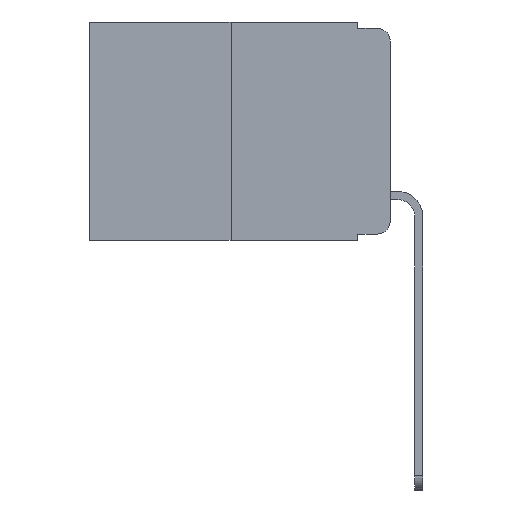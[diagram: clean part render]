
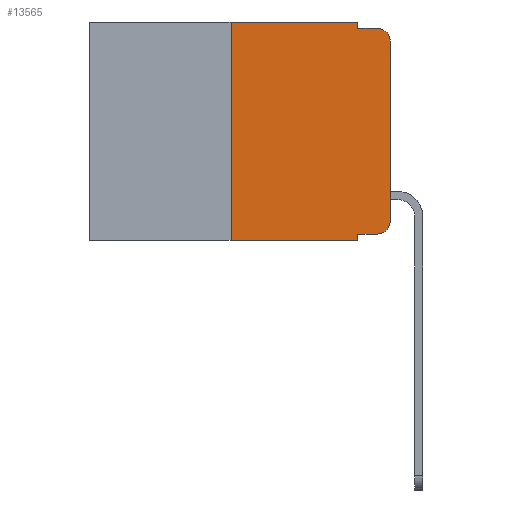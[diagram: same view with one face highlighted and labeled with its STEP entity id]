
A CAD part, left-side view. The second image highlights one B-rep face of the part: STEP entity #13565.
In plain terms, the highlighted planar face has unit normal (-1, 0, 0).
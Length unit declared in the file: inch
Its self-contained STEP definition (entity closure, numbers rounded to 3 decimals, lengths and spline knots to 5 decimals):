
#200 = EDGE_CURVE ( 'NONE', #16127, #12998, #8034, .T. ) ;
#222 = AXIS2_PLACEMENT_3D ( 'NONE', #17483, #13015, #17306 ) ;
#324 = ORIENTED_EDGE ( 'NONE', *, *, #8914, .T. ) ;
#459 = VECTOR ( 'NONE', #4900, 39.37008 ) ;
#764 = ORIENTED_EDGE ( 'NONE', *, *, #16925, .F. ) ;
#1282 = EDGE_CURVE ( 'NONE', #5609, #7590, #9548, .T. ) ;
#1350 = DIRECTION ( 'NONE',  ( 0., 0., -1. ) ) ;
#1611 = ORIENTED_EDGE ( 'NONE', *, *, #16746, .F. ) ;
#1637 = CARTESIAN_POINT ( 'NONE',  ( 0., 0.02, -0.313 ) ) ;
#1811 = VECTOR ( 'NONE', #4530, 39.37008 ) ;
#1812 = ORIENTED_EDGE ( 'NONE', *, *, #15690, .F. ) ;
#2113 = CIRCLE ( 'NONE', #18376, 0.02 ) ;
#3090 = VECTOR ( 'NONE', #7911, 39.37008 ) ;
#3169 = PLANE ( 'NONE',  #16164 ) ;
#3300 = EDGE_CURVE ( 'NONE', #13375, #14258, #11208, .T. ) ;
#3747 = VECTOR ( 'NONE', #1350, 39.37008 ) ;
#4145 = EDGE_CURVE ( 'NONE', #5609, #15441, #12513, .T. ) ;
#4530 = DIRECTION ( 'NONE',  ( 0., -1., 0. ) ) ;
#4900 = DIRECTION ( 'NONE',  ( 0., 0., 1. ) ) ;
#5467 = DIRECTION ( 'NONE',  ( 0., -1., 0. ) ) ;
#5485 = DIRECTION ( 'NONE',  ( 0., -1., 0. ) ) ;
#5609 = VERTEX_POINT ( 'NONE', #14676 ) ;
#5789 = CARTESIAN_POINT ( 'NONE',  ( 0., 0.051, -0.333 ) ) ;
#5985 = VERTEX_POINT ( 'NONE', #17091 ) ;
#6039 = CIRCLE ( 'NONE', #222, 0.02 ) ;
#6047 = CARTESIAN_POINT ( 'NONE',  ( 0., 0.473, 0. ) ) ;
#6854 = FACE_OUTER_BOUND ( 'NONE', #14925, .T. ) ;
#7193 = ORIENTED_EDGE ( 'NONE', *, *, #200, .T. ) ;
#7463 = ORIENTED_EDGE ( 'NONE', *, *, #4145, .T. ) ;
#7585 = CARTESIAN_POINT ( 'NONE',  ( 0., 0.25, 0. ) ) ;
#7590 = VERTEX_POINT ( 'NONE', #17943 ) ;
#7911 = DIRECTION ( 'NONE',  ( 0., -1., 0. ) ) ;
#8034 = LINE ( 'NONE', #16180, #459 ) ;
#8217 = VECTOR ( 'NONE', #11835, 39.37008 ) ;
#8445 = LINE ( 'NONE', #9388, #3090 ) ;
#8742 = CARTESIAN_POINT ( 'NONE',  ( 0., 0.051, -0.333 ) ) ;
#8914 = EDGE_CURVE ( 'NONE', #14258, #16127, #2113, .T. ) ;
#8921 = DIRECTION ( 'NONE',  ( 0., 0., -1. ) ) ;
#9120 = CARTESIAN_POINT ( 'NONE',  ( 0., 0., -0.03 ) ) ;
#9388 = CARTESIAN_POINT ( 'NONE',  ( 0., 0.051, -0.01 ) ) ;
#9548 = LINE ( 'NONE', #7585, #8217 ) ;
#10880 = VERTEX_POINT ( 'NONE', #17866 ) ;
#11109 = EDGE_CURVE ( 'NONE', #12998, #5985, #6039, .T. ) ;
#11208 = LINE ( 'NONE', #5789, #1811 ) ;
#11218 = CARTESIAN_POINT ( 'NONE',  ( 0., 0.473, -0.343 ) ) ;
#11639 = ORIENTED_EDGE ( 'NONE', *, *, #3300, .T. ) ;
#11835 = DIRECTION ( 'NONE',  ( 0., 0., 1. ) ) ;
#12057 = CARTESIAN_POINT ( 'NONE',  ( 0., 0., -0.313 ) ) ;
#12318 = DIRECTION ( 'NONE',  ( 0., 0., -1. ) ) ;
#12513 = LINE ( 'NONE', #11218, #18105 ) ;
#12761 = VECTOR ( 'NONE', #12318, 39.37008 ) ;
#12998 = VERTEX_POINT ( 'NONE', #9120 ) ;
#13015 = DIRECTION ( 'NONE',  ( -1., 0., 0. ) ) ;
#13069 = DIRECTION ( 'NONE',  ( -1., 0., 0. ) ) ;
#13155 = LINE ( 'NONE', #18465, #3747 ) ;
#13375 = VERTEX_POINT ( 'NONE', #8742 ) ;
#13565 = ADVANCED_FACE ( 'NONE', ( #6854 ), #3169, .F. ) ;
#14181 = CARTESIAN_POINT ( 'NONE',  ( 0., 0.473, 0. ) ) ;
#14258 = VERTEX_POINT ( 'NONE', #18322 ) ;
#14495 = DIRECTION ( 'NONE',  ( 0., 0., -1. ) ) ;
#14676 = CARTESIAN_POINT ( 'NONE',  ( 0., 0.25, -0.343 ) ) ;
#14694 = CARTESIAN_POINT ( 'NONE',  ( 0., 0.051, -0.343 ) ) ;
#14738 = ORIENTED_EDGE ( 'NONE', *, *, #11109, .T. ) ;
#14779 = DIRECTION ( 'NONE',  ( 1., 0., 0. ) ) ;
#14925 = EDGE_LOOP ( 'NONE', ( #7193, #14738, #1611, #764, #16896, #18173, #7463, #1812, #11639, #324 ) ) ;
#15298 = CARTESIAN_POINT ( 'NONE',  ( 0., 0.051, 0. ) ) ;
#15441 = VERTEX_POINT ( 'NONE', #14694 ) ;
#15690 = EDGE_CURVE ( 'NONE', #13375, #15441, #17435, .T. ) ;
#15807 = EDGE_CURVE ( 'NONE', #7590, #17962, #17214, .T. ) ;
#15880 = VECTOR ( 'NONE', #5485, 39.37008 ) ;
#16127 = VERTEX_POINT ( 'NONE', #12057 ) ;
#16164 = AXIS2_PLACEMENT_3D ( 'NONE', #6047, #14779, #8921 ) ;
#16180 = CARTESIAN_POINT ( 'NONE',  ( 0., 0., 0. ) ) ;
#16746 = EDGE_CURVE ( 'NONE', #10880, #5985, #8445, .T. ) ;
#16896 = ORIENTED_EDGE ( 'NONE', *, *, #15807, .F. ) ;
#16925 = EDGE_CURVE ( 'NONE', #17962, #10880, #13155, .T. ) ;
#17091 = CARTESIAN_POINT ( 'NONE',  ( 0., 0.02, -0.01 ) ) ;
#17214 = LINE ( 'NONE', #14181, #15880 ) ;
#17306 = DIRECTION ( 'NONE',  ( 0., 0., -1. ) ) ;
#17435 = LINE ( 'NONE', #15298, #12761 ) ;
#17483 = CARTESIAN_POINT ( 'NONE',  ( 0., 0.02, -0.03 ) ) ;
#17726 = CARTESIAN_POINT ( 'NONE',  ( 0., 0.051, 0. ) ) ;
#17866 = CARTESIAN_POINT ( 'NONE',  ( 0., 0.051, -0.01 ) ) ;
#17943 = CARTESIAN_POINT ( 'NONE',  ( 0., 0.25, 0. ) ) ;
#17962 = VERTEX_POINT ( 'NONE', #17726 ) ;
#18105 = VECTOR ( 'NONE', #5467, 39.37008 ) ;
#18173 = ORIENTED_EDGE ( 'NONE', *, *, #1282, .F. ) ;
#18322 = CARTESIAN_POINT ( 'NONE',  ( 0., 0.02, -0.333 ) ) ;
#18376 = AXIS2_PLACEMENT_3D ( 'NONE', #1637, #13069, #14495 ) ;
#18465 = CARTESIAN_POINT ( 'NONE',  ( 0., 0.051, 0. ) ) ;
